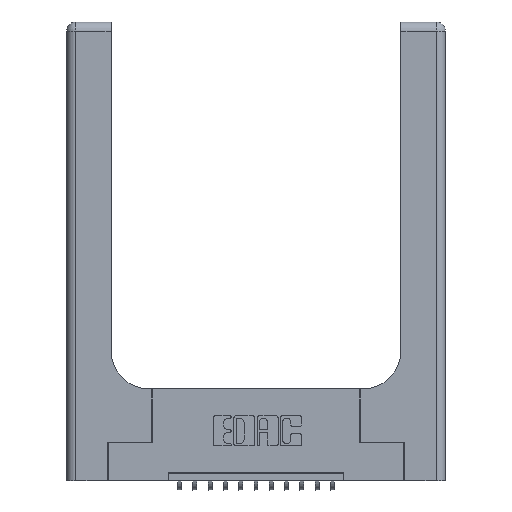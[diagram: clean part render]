
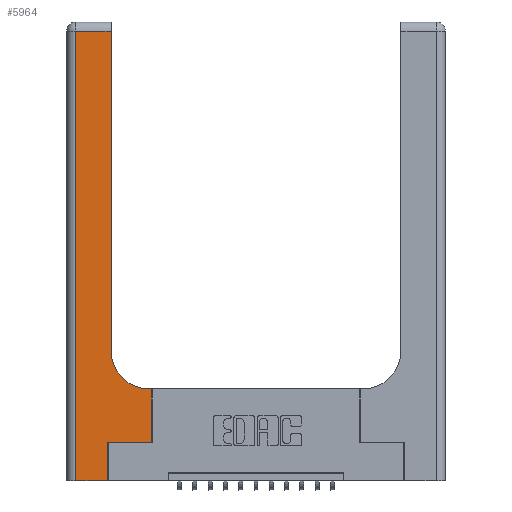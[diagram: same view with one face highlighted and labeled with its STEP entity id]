
A CAD part, top view. The second image highlights one B-rep face of the part: STEP entity #5964.
In plain terms, the highlighted planar face has unit normal (0, 0, 1).
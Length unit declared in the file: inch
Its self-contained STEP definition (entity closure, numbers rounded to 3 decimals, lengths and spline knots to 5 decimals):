
#41 = VECTOR ( 'NONE', #6102, 39.37008 ) ;
#531 = CARTESIAN_POINT ( 'NONE',  ( 0.5585, 0.25, 0.37 ) ) ;
#1111 = CARTESIAN_POINT ( 'NONE',  ( 0.2915, 0.6, 0.37 ) ) ;
#1165 = CARTESIAN_POINT ( 'NONE',  ( 0., 3., 0.37 ) ) ;
#1287 = AXIS2_PLACEMENT_3D ( 'NONE', #13781, #8328, #8514 ) ;
#2045 = VERTEX_POINT ( 'NONE', #11270 ) ;
#2753 = ORIENTED_EDGE ( 'NONE', *, *, #9708, .T. ) ;
#3891 = CARTESIAN_POINT ( 'NONE',  ( 0.2915, 0.85, 0.37 ) ) ;
#3963 = PLANE ( 'NONE',  #11031 ) ;
#4046 = CARTESIAN_POINT ( 'NONE',  ( 0.269, 0.25, 0.37 ) ) ;
#4094 = VECTOR ( 'NONE', #16194, 39.37008 ) ;
#4142 = ORIENTED_EDGE ( 'NONE', *, *, #13062, .T. ) ;
#4187 = DIRECTION ( 'NONE',  ( 1., 0., 0. ) ) ;
#4580 = DIRECTION ( 'NONE',  ( 0., -1., 0. ) ) ;
#5576 = CARTESIAN_POINT ( 'NONE',  ( 0.5585, 0.25, 0.37 ) ) ;
#5614 = CARTESIAN_POINT ( 'NONE',  ( 0., 0., 0.37 ) ) ;
#5922 = CARTESIAN_POINT ( 'NONE',  ( 0.269, 0.25, 0.37 ) ) ;
#5964 = ADVANCED_FACE ( 'NONE', ( #10345 ), #3963, .F. ) ;
#6102 = DIRECTION ( 'NONE',  ( -1., 0., 0. ) ) ;
#6143 = EDGE_CURVE ( 'NONE', #14840, #14793, #14389, .T. ) ;
#6365 = VERTEX_POINT ( 'NONE', #7687 ) ;
#6575 = CARTESIAN_POINT ( 'NONE',  ( 0.2915, 3., 0.37 ) ) ;
#6914 = DIRECTION ( 'NONE',  ( 0., 1., 0. ) ) ;
#7152 = EDGE_CURVE ( 'NONE', #15042, #16980, #9471, .T. ) ;
#7340 = VECTOR ( 'NONE', #10027, 39.37008 ) ;
#7362 = DIRECTION ( 'NONE',  ( 0., 1., 0. ) ) ;
#7648 = CARTESIAN_POINT ( 'NONE',  ( 0.06, 0., 0.37 ) ) ;
#7687 = CARTESIAN_POINT ( 'NONE',  ( 0.5585, 0.6, 0.37 ) ) ;
#7762 = LINE ( 'NONE', #6575, #4094 ) ;
#8221 = EDGE_LOOP ( 'NONE', ( #14912, #16649, #2753, #11816, #11417, #4142, #11039, #16510, #8472 ) ) ;
#8328 = DIRECTION ( 'NONE',  ( 0., 0., -1. ) ) ;
#8472 = ORIENTED_EDGE ( 'NONE', *, *, #6143, .T. ) ;
#8514 = DIRECTION ( 'NONE',  ( 1., 0., 0. ) ) ;
#9402 = CARTESIAN_POINT ( 'NONE',  ( 0.5415, 0.6, 0.37 ) ) ;
#9471 = LINE ( 'NONE', #15257, #16347 ) ;
#9685 = VECTOR ( 'NONE', #4187, 39.37008 ) ;
#9708 = EDGE_CURVE ( 'NONE', #2045, #10234, #15681, .T. ) ;
#10027 = DIRECTION ( 'NONE',  ( -1., 0., 0. ) ) ;
#10234 = VERTEX_POINT ( 'NONE', #7648 ) ;
#10345 = FACE_OUTER_BOUND ( 'NONE', #8221, .T. ) ;
#10526 = LINE ( 'NONE', #12928, #41 ) ;
#10726 = DIRECTION ( 'NONE',  ( 0., 0., -1. ) ) ;
#11031 = AXIS2_PLACEMENT_3D ( 'NONE', #1165, #10726, #16272 ) ;
#11039 = ORIENTED_EDGE ( 'NONE', *, *, #11950, .T. ) ;
#11172 = LINE ( 'NONE', #1111, #7340 ) ;
#11270 = CARTESIAN_POINT ( 'NONE',  ( 0.06, 2.94, 0.37 ) ) ;
#11355 = CARTESIAN_POINT ( 'NONE',  ( 0.2915, 2.94, 0.37 ) ) ;
#11417 = ORIENTED_EDGE ( 'NONE', *, *, #7152, .T. ) ;
#11434 = CARTESIAN_POINT ( 'NONE',  ( 0.06, 3., 0.37 ) ) ;
#11507 = LINE ( 'NONE', #5576, #12988 ) ;
#11680 = LINE ( 'NONE', #5922, #13812 ) ;
#11816 = ORIENTED_EDGE ( 'NONE', *, *, #14919, .T. ) ;
#11950 = EDGE_CURVE ( 'NONE', #12431, #6365, #11507, .T. ) ;
#12022 = VECTOR ( 'NONE', #4580, 39.37008 ) ;
#12431 = VERTEX_POINT ( 'NONE', #531 ) ;
#12565 = CARTESIAN_POINT ( 'NONE',  ( 0.269, 0., 0.37 ) ) ;
#12928 = CARTESIAN_POINT ( 'NONE',  ( 0., 2.94, 0.37 ) ) ;
#12988 = VECTOR ( 'NONE', #6914, 39.37008 ) ;
#13062 = EDGE_CURVE ( 'NONE', #16980, #12431, #11680, .T. ) ;
#13489 = VERTEX_POINT ( 'NONE', #11355 ) ;
#13781 = CARTESIAN_POINT ( 'NONE',  ( 0.5415, 0.85, 0.37 ) ) ;
#13812 = VECTOR ( 'NONE', #17138, 39.37008 ) ;
#14389 = CIRCLE ( 'NONE', #1287, 0.25 ) ;
#14747 = EDGE_CURVE ( 'NONE', #6365, #14840, #11172, .T. ) ;
#14793 = VERTEX_POINT ( 'NONE', #3891 ) ;
#14840 = VERTEX_POINT ( 'NONE', #9402 ) ;
#14912 = ORIENTED_EDGE ( 'NONE', *, *, #15419, .T. ) ;
#14919 = EDGE_CURVE ( 'NONE', #10234, #15042, #15709, .T. ) ;
#15042 = VERTEX_POINT ( 'NONE', #12565 ) ;
#15160 = EDGE_CURVE ( 'NONE', #13489, #2045, #10526, .T. ) ;
#15257 = CARTESIAN_POINT ( 'NONE',  ( 0.269, 0., 0.37 ) ) ;
#15419 = EDGE_CURVE ( 'NONE', #14793, #13489, #7762, .T. ) ;
#15681 = LINE ( 'NONE', #11434, #12022 ) ;
#15709 = LINE ( 'NONE', #5614, #9685 ) ;
#16194 = DIRECTION ( 'NONE',  ( 0., 1., 0. ) ) ;
#16272 = DIRECTION ( 'NONE',  ( -1., 0., 0. ) ) ;
#16347 = VECTOR ( 'NONE', #7362, 39.37008 ) ;
#16510 = ORIENTED_EDGE ( 'NONE', *, *, #14747, .T. ) ;
#16649 = ORIENTED_EDGE ( 'NONE', *, *, #15160, .T. ) ;
#16980 = VERTEX_POINT ( 'NONE', #4046 ) ;
#17138 = DIRECTION ( 'NONE',  ( 1., 0., 0. ) ) ;
